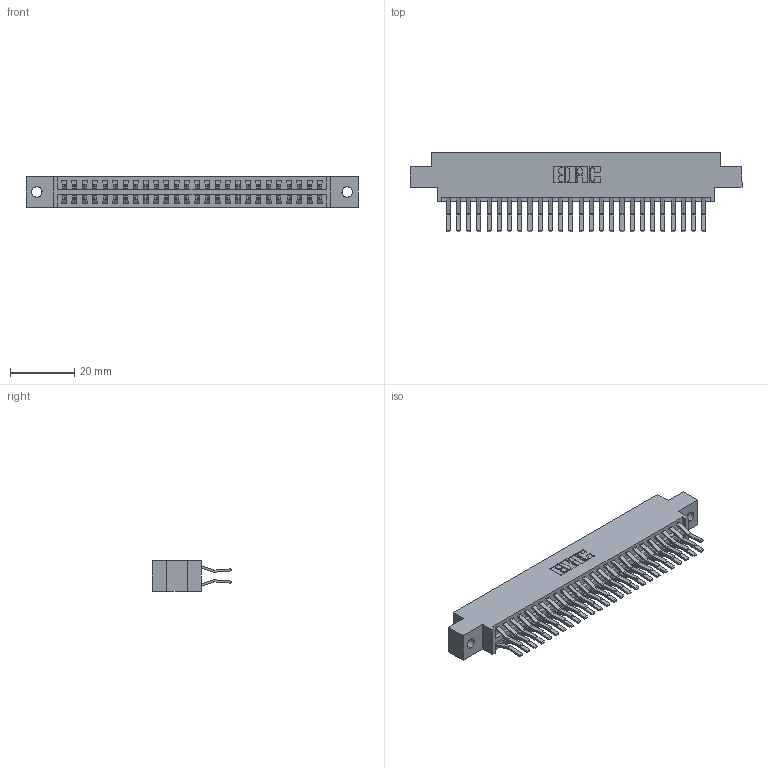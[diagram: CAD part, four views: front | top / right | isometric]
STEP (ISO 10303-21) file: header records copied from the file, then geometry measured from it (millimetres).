
FILE_DESCRIPTION (( 'STEP AP203' ), '1' );
FILE_NAME ('396-052-560-802.STEP', '2018-09-08T07:15:54', ( '' ), ( '' ), 'SwSTEP 2.0', 'SolidWorks 2016', '' );
FILE_SCHEMA (( 'CONFIG_CONTROL_DESIGN' ));
Length unit declared in the file: inch
Products named in the file (3): 346 Part_0.170 Offset - 0.128 Dia; 345-292-001_560 Tail; 396-052-560-802
Assembly tree (53 placements, depth 2):
  396-052-560-802
    346 Part_0.170 Offset - 0.128 Dia
    345-292-001_560 Tail  x52
Bounding box: 103.12 x 24.78 x 9.4 mm (x, y, z)
Volume: 10081.1 mm3; surface area: 14425.4 mm2
Topology: 53 solids, 53 shells, 2934 faces, 8713 edges, 5738 vertices
Faces by surface type: plane 1900, cylinder 1034
Entity records: 19345 total; most frequent: CARTESIAN_POINT 3212, ORIENTED_EDGE 3146, DIRECTION 2885, EDGE_CURVE 1573, LINE 1333, VECTOR 1333, VERTEX_POINT 1046, AXIS2_PLACEMENT_3D 776
